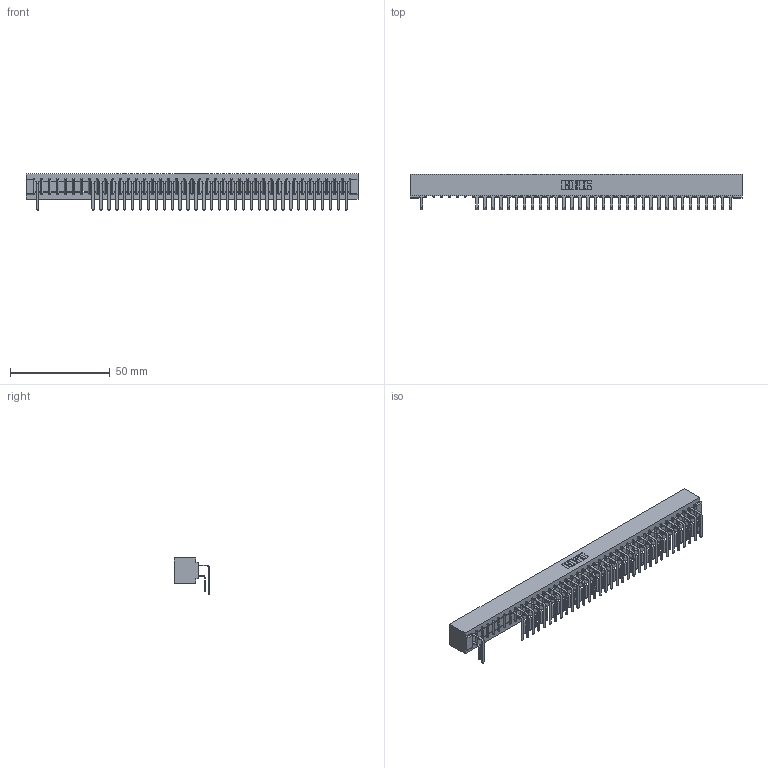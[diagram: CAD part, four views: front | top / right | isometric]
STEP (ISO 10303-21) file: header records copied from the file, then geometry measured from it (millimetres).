
FILE_DESCRIPTION (( 'STEP AP203' ), '1' );
FILE_NAME ('307-040-559-101.STEP', '2018-08-05T13:58:35', ( '' ), ( '' ), 'SwSTEP 2.0', 'SolidWorks 2016', '' );
FILE_SCHEMA (( 'CONFIG_CONTROL_DESIGN' ));
Length unit declared in the file: inch
Products named in the file (4): 307 Part_No Mounting Lugs; 307-290-001_558 559 - 1 (Single); 307-290-001_559 - 2 (Single); 307-040-559-101
Assembly tree (68 placements, depth 2):
  307-040-559-101
    307 Part_No Mounting Lugs
    307-290-001_558 559 - 1 (Single)  x33
    307-290-001_559 - 2 (Single)  x34
Bounding box: 166.37 x 17.69 x 18.07 mm (x, y, z)
Volume: 18355.2 mm3; surface area: 23369.2 mm2
Topology: 68 solids, 68 shells, 3631 faces, 10229 edges, 6618 vertices
Faces by surface type: plane 2355, cylinder 1194, sphere 82
Entity records: 36571 total; most frequent: CARTESIAN_POINT 6037, ORIENTED_EDGE 5994, DIRECTION 5899, EDGE_CURVE 2997, VECTOR 2299, LINE 2299, VERTEX_POINT 1938, AXIS2_PLACEMENT_3D 1800
